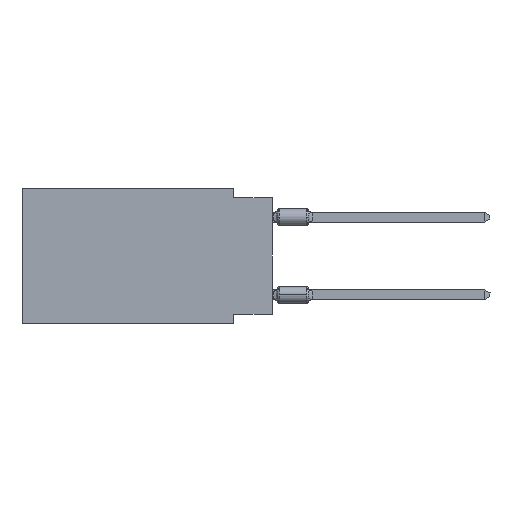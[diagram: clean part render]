
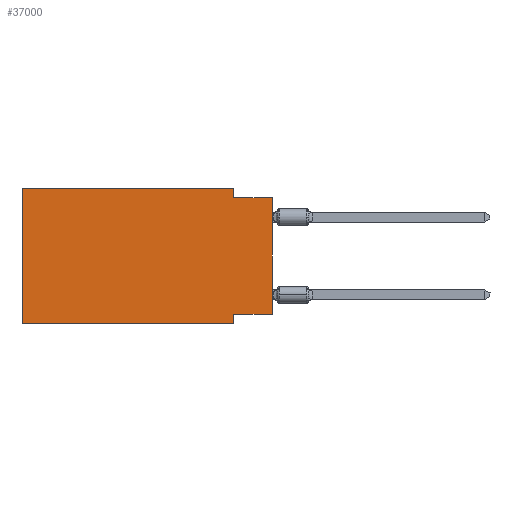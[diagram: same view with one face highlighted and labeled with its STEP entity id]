
A CAD part, left-side view. The second image highlights one B-rep face of the part: STEP entity #37000.
In plain terms, the highlighted planar face has unit normal (-1, 0, 0).
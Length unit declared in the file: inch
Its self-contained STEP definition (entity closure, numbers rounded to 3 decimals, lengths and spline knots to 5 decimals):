
#427 = ORIENTED_EDGE ( 'NONE', *, *, #4933, .F. ) ;
#1286 = VERTEX_POINT ( 'NONE', #57109 ) ;
#1797 = CARTESIAN_POINT ( 'NONE',  ( 0., 0.1, 0. ) ) ;
#2121 = CARTESIAN_POINT ( 'NONE',  ( 0., 0., -0.025 ) ) ;
#2834 = EDGE_CURVE ( 'NONE', #38839, #45412, #55329, .T. ) ;
#3254 = ORIENTED_EDGE ( 'NONE', *, *, #10151, .F. ) ;
#3582 = VECTOR ( 'NONE', #25109, 39.37008 ) ;
#3824 = LINE ( 'NONE', #4169, #3582 ) ;
#4038 = LINE ( 'NONE', #18694, #51682 ) ;
#4169 = CARTESIAN_POINT ( 'NONE',  ( 0., 0.1, -0.35 ) ) ;
#4672 = VECTOR ( 'NONE', #65827, 39.37008 ) ;
#4933 = EDGE_CURVE ( 'NONE', #58732, #9241, #61685, .T. ) ;
#5690 = VECTOR ( 'NONE', #43663, 39.37008 ) ;
#5918 = EDGE_CURVE ( 'NONE', #38839, #56392, #7646, .T. ) ;
#7562 = CARTESIAN_POINT ( 'NONE',  ( 0., 0., 0. ) ) ;
#7646 = LINE ( 'NONE', #29256, #4672 ) ;
#7991 = PLANE ( 'NONE',  #31639 ) ;
#8917 = DIRECTION ( 'NONE',  ( 0., 0., -1. ) ) ;
#9241 = VERTEX_POINT ( 'NONE', #1797 ) ;
#9608 = ORIENTED_EDGE ( 'NONE', *, *, #54627, .F. ) ;
#10151 = EDGE_CURVE ( 'NONE', #9241, #1286, #4038, .T. ) ;
#11213 = ORIENTED_EDGE ( 'NONE', *, *, #5918, .F. ) ;
#14172 = ORIENTED_EDGE ( 'NONE', *, *, #2834, .T. ) ;
#16442 = DIRECTION ( 'NONE',  ( 0., 0., 1. ) ) ;
#17497 = CARTESIAN_POINT ( 'NONE',  ( 0., 0.645, -0.35 ) ) ;
#17997 = VECTOR ( 'NONE', #50073, 39.37008 ) ;
#18694 = CARTESIAN_POINT ( 'NONE',  ( 0., 0.1, 0. ) ) ;
#18803 = CARTESIAN_POINT ( 'NONE',  ( 0., 0.645, 0. ) ) ;
#21061 = CARTESIAN_POINT ( 'NONE',  ( 0., 0.645, -0.35 ) ) ;
#25109 = DIRECTION ( 'NONE',  ( 0., 0., -1. ) ) ;
#29140 = CARTESIAN_POINT ( 'NONE',  ( 0., 0., -0.025 ) ) ;
#29256 = CARTESIAN_POINT ( 'NONE',  ( 0., 0., -0.325 ) ) ;
#29644 = FACE_OUTER_BOUND ( 'NONE', #62663, .T. ) ;
#29845 = ORIENTED_EDGE ( 'NONE', *, *, #66339, .F. ) ;
#30464 = VECTOR ( 'NONE', #39733, 39.37008 ) ;
#31639 = AXIS2_PLACEMENT_3D ( 'NONE', #45614, #34472, #40773 ) ;
#33072 = VERTEX_POINT ( 'NONE', #67604 ) ;
#34151 = EDGE_CURVE ( 'NONE', #61880, #33072, #38100, .T. ) ;
#34472 = DIRECTION ( 'NONE',  ( 1., 0., 0. ) ) ;
#34842 = CARTESIAN_POINT ( 'NONE',  ( 0., 0.645, 0. ) ) ;
#36779 = CARTESIAN_POINT ( 'NONE',  ( 0., 0.1, -0.325 ) ) ;
#36971 = CARTESIAN_POINT ( 'NONE',  ( 0., 0.645, 0. ) ) ;
#37000 = ADVANCED_FACE ( 'NONE', ( #29644 ), #7991, .F. ) ;
#38100 = LINE ( 'NONE', #21061, #5690 ) ;
#38839 = VERTEX_POINT ( 'NONE', #65515 ) ;
#39733 = DIRECTION ( 'NONE',  ( 0., -1., 0. ) ) ;
#40773 = DIRECTION ( 'NONE',  ( 0., 0., -1. ) ) ;
#43663 = DIRECTION ( 'NONE',  ( 0., -1., 0. ) ) ;
#45412 = VERTEX_POINT ( 'NONE', #29140 ) ;
#45614 = CARTESIAN_POINT ( 'NONE',  ( 0., 0.645, 0. ) ) ;
#50073 = DIRECTION ( 'NONE',  ( 0., 0., 1. ) ) ;
#50541 = VECTOR ( 'NONE', #16442, 39.37008 ) ;
#51682 = VECTOR ( 'NONE', #8917, 39.37008 ) ;
#54627 = EDGE_CURVE ( 'NONE', #61880, #58732, #58253, .T. ) ;
#54826 = VECTOR ( 'NONE', #55803, 39.37008 ) ;
#55329 = LINE ( 'NONE', #7562, #17997 ) ;
#55803 = DIRECTION ( 'NONE',  ( 0., -1., 0. ) ) ;
#56392 = VERTEX_POINT ( 'NONE', #36779 ) ;
#57109 = CARTESIAN_POINT ( 'NONE',  ( 0., 0.1, -0.025 ) ) ;
#58253 = LINE ( 'NONE', #36971, #50541 ) ;
#58732 = VERTEX_POINT ( 'NONE', #34842 ) ;
#61046 = LINE ( 'NONE', #2121, #54826 ) ;
#61685 = LINE ( 'NONE', #18803, #30464 ) ;
#61880 = VERTEX_POINT ( 'NONE', #17497 ) ;
#62663 = EDGE_LOOP ( 'NONE', ( #14172, #29845, #3254, #427, #9608, #67730, #68049, #11213 ) ) ;
#65515 = CARTESIAN_POINT ( 'NONE',  ( 0., 0., -0.325 ) ) ;
#65827 = DIRECTION ( 'NONE',  ( 0., 1., 0. ) ) ;
#66339 = EDGE_CURVE ( 'NONE', #1286, #45412, #61046, .T. ) ;
#67604 = CARTESIAN_POINT ( 'NONE',  ( 0., 0.1, -0.35 ) ) ;
#67730 = ORIENTED_EDGE ( 'NONE', *, *, #34151, .T. ) ;
#68049 = ORIENTED_EDGE ( 'NONE', *, *, #68582, .F. ) ;
#68582 = EDGE_CURVE ( 'NONE', #56392, #33072, #3824, .T. ) ;
